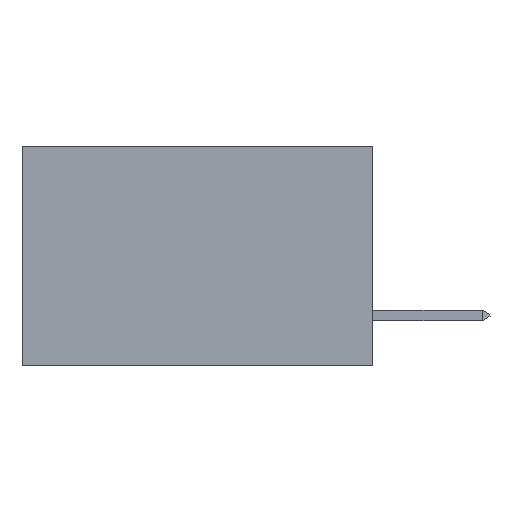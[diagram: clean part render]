
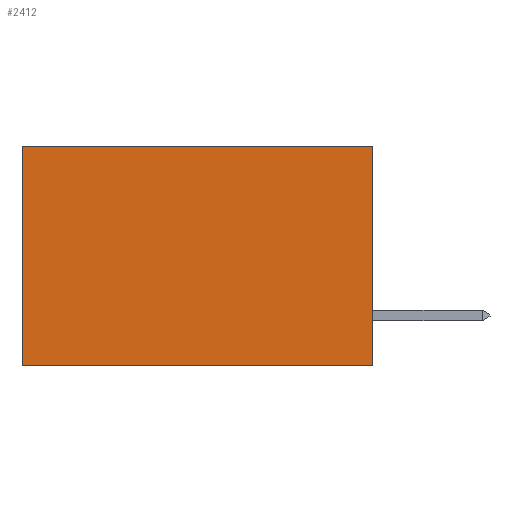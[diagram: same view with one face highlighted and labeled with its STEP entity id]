
A CAD part, left-side view. The second image highlights one B-rep face of the part: STEP entity #2412.
In plain terms, the highlighted planar face has unit normal (-1, 0, 0).
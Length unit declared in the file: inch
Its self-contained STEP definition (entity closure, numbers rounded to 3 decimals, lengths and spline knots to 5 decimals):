
#96 = ORIENTED_EDGE ( 'NONE', *, *, #5063, .F. ) ;
#98 = EDGE_CURVE ( 'NONE', #960, #8671, #5756, .T. ) ;
#480 = FACE_OUTER_BOUND ( 'NONE', #7415, .T. ) ;
#596 = VECTOR ( 'NONE', #797, 39.37008 ) ;
#609 = AXIS2_PLACEMENT_3D ( 'NONE', #5354, #7709, #6354 ) ;
#797 = DIRECTION ( 'NONE',  ( 0., 1., 0. ) ) ;
#873 = CARTESIAN_POINT ( 'NONE',  ( 0.277, 0.59, -0.37 ) ) ;
#960 = VERTEX_POINT ( 'NONE', #3943 ) ;
#1879 = ORIENTED_EDGE ( 'NONE', *, *, #98, .T. ) ;
#2412 = ADVANCED_FACE ( 'NONE', ( #480 ), #7053, .F. ) ;
#2715 = VECTOR ( 'NONE', #2865, 39.37008 ) ;
#2865 = DIRECTION ( 'NONE',  ( 0., 0., -1. ) ) ;
#3045 = CARTESIAN_POINT ( 'NONE',  ( 0.277, 0., -0.37 ) ) ;
#3943 = CARTESIAN_POINT ( 'NONE',  ( 0.277, 0.59, 0. ) ) ;
#4140 = ORIENTED_EDGE ( 'NONE', *, *, #5705, .F. ) ;
#5035 = VERTEX_POINT ( 'NONE', #6966 ) ;
#5063 = EDGE_CURVE ( 'NONE', #7829, #8671, #6295, .T. ) ;
#5354 = CARTESIAN_POINT ( 'NONE',  ( 0.277, 0., -0.37 ) ) ;
#5429 = CARTESIAN_POINT ( 'NONE',  ( 0.277, 0., -0.37 ) ) ;
#5705 = EDGE_CURVE ( 'NONE', #5035, #7829, #8595, .T. ) ;
#5756 = LINE ( 'NONE', #8208, #9138 ) ;
#6295 = LINE ( 'NONE', #6763, #7893 ) ;
#6354 = DIRECTION ( 'NONE',  ( 0., 0., -1. ) ) ;
#6362 = EDGE_CURVE ( 'NONE', #5035, #960, #6487, .T. ) ;
#6487 = LINE ( 'NONE', #8877, #596 ) ;
#6707 = DIRECTION ( 'NONE',  ( 0., 1., 0. ) ) ;
#6763 = CARTESIAN_POINT ( 'NONE',  ( 0.277, 0., -0.37 ) ) ;
#6966 = CARTESIAN_POINT ( 'NONE',  ( 0.277, 0., 0. ) ) ;
#7008 = DIRECTION ( 'NONE',  ( 0., 0., -1. ) ) ;
#7053 = PLANE ( 'NONE',  #609 ) ;
#7415 = EDGE_LOOP ( 'NONE', ( #1879, #96, #4140, #7858 ) ) ;
#7709 = DIRECTION ( 'NONE',  ( 1., 0., 0. ) ) ;
#7829 = VERTEX_POINT ( 'NONE', #5429 ) ;
#7858 = ORIENTED_EDGE ( 'NONE', *, *, #6362, .T. ) ;
#7893 = VECTOR ( 'NONE', #6707, 39.37008 ) ;
#8208 = CARTESIAN_POINT ( 'NONE',  ( 0.277, 0.59, -0.37 ) ) ;
#8595 = LINE ( 'NONE', #3045, #2715 ) ;
#8671 = VERTEX_POINT ( 'NONE', #873 ) ;
#8877 = CARTESIAN_POINT ( 'NONE',  ( 0.277, 0., 0. ) ) ;
#9138 = VECTOR ( 'NONE', #7008, 39.37008 ) ;
